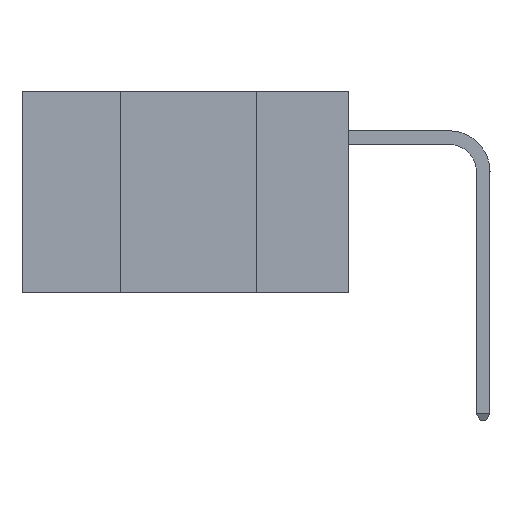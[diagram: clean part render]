
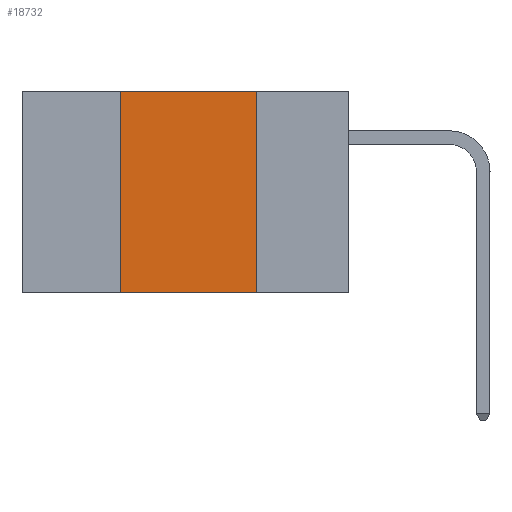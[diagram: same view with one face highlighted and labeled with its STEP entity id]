
A CAD part, left-side view. The second image highlights one B-rep face of the part: STEP entity #18732.
In plain terms, the highlighted planar face has unit normal (-1, 0, 0).
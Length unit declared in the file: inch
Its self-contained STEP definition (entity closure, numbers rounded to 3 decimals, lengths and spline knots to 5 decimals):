
#55 = DIRECTION ( 'NONE',  ( 1., 0., 0. ) ) ;
#493 = CARTESIAN_POINT ( 'NONE',  ( 0., 0.6, 0. ) ) ;
#977 = VECTOR ( 'NONE', #981, 39.37008 ) ;
#981 = DIRECTION ( 'NONE',  ( 0., -1., 0. ) ) ;
#2071 = ORIENTED_EDGE ( 'NONE', *, *, #12484, .T. ) ;
#2368 = LINE ( 'NONE', #493, #30756 ) ;
#2394 = VERTEX_POINT ( 'NONE', #10128 ) ;
#2610 = LINE ( 'NONE', #17393, #25899 ) ;
#9177 = CARTESIAN_POINT ( 'NONE',  ( 0., 0.6, 0. ) ) ;
#10128 = CARTESIAN_POINT ( 'NONE',  ( 0., 0.17, 0. ) ) ;
#10437 = EDGE_CURVE ( 'NONE', #2394, #26907, #29597, .T. ) ;
#12484 = EDGE_CURVE ( 'NONE', #20367, #26907, #25254, .T. ) ;
#12690 = CARTESIAN_POINT ( 'NONE',  ( 0., 0.17, 0. ) ) ;
#13235 = CARTESIAN_POINT ( 'NONE',  ( 0., 0.6, -0.37 ) ) ;
#14184 = EDGE_CURVE ( 'NONE', #37811, #2394, #2368, .T. ) ;
#17393 = CARTESIAN_POINT ( 'NONE',  ( 0., 0.42, 0. ) ) ;
#18362 = PLANE ( 'NONE',  #29888 ) ;
#18365 = CARTESIAN_POINT ( 'NONE',  ( 0., 0.17, -0.37 ) ) ;
#18732 = ADVANCED_FACE ( 'NONE', ( #37384 ), #18362, .F. ) ;
#20367 = VERTEX_POINT ( 'NONE', #33963 ) ;
#20463 = DIRECTION ( 'NONE',  ( 0., 0., 1. ) ) ;
#20643 = EDGE_CURVE ( 'NONE', #20367, #37811, #2610, .T. ) ;
#21386 = DIRECTION ( 'NONE',  ( 0., 0., -1. ) ) ;
#21631 = ORIENTED_EDGE ( 'NONE', *, *, #10437, .F. ) ;
#24919 = EDGE_LOOP ( 'NONE', ( #21631, #31422, #32368, #2071 ) ) ;
#25254 = LINE ( 'NONE', #13235, #977 ) ;
#25899 = VECTOR ( 'NONE', #20463, 39.37008 ) ;
#26907 = VERTEX_POINT ( 'NONE', #18365 ) ;
#29597 = LINE ( 'NONE', #12690, #30530 ) ;
#29888 = AXIS2_PLACEMENT_3D ( 'NONE', #9177, #55, #21386 ) ;
#30530 = VECTOR ( 'NONE', #30629, 39.37008 ) ;
#30629 = DIRECTION ( 'NONE',  ( 0., 0., -1. ) ) ;
#30756 = VECTOR ( 'NONE', #30798, 39.37008 ) ;
#30798 = DIRECTION ( 'NONE',  ( 0., -1., 0. ) ) ;
#31422 = ORIENTED_EDGE ( 'NONE', *, *, #14184, .F. ) ;
#32368 = ORIENTED_EDGE ( 'NONE', *, *, #20643, .F. ) ;
#33391 = CARTESIAN_POINT ( 'NONE',  ( 0., 0.42, 0. ) ) ;
#33963 = CARTESIAN_POINT ( 'NONE',  ( 0., 0.42, -0.37 ) ) ;
#37384 = FACE_OUTER_BOUND ( 'NONE', #24919, .T. ) ;
#37811 = VERTEX_POINT ( 'NONE', #33391 ) ;
